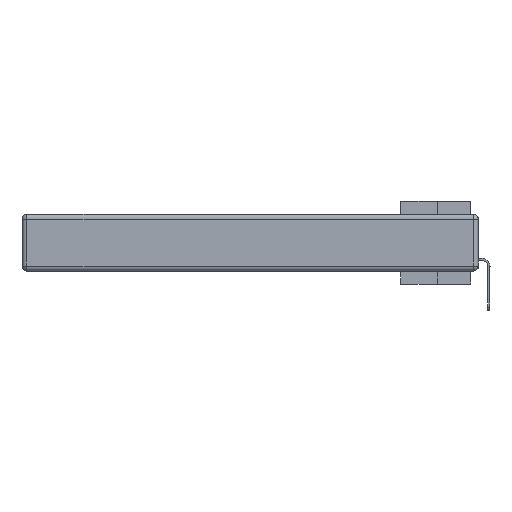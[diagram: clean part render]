
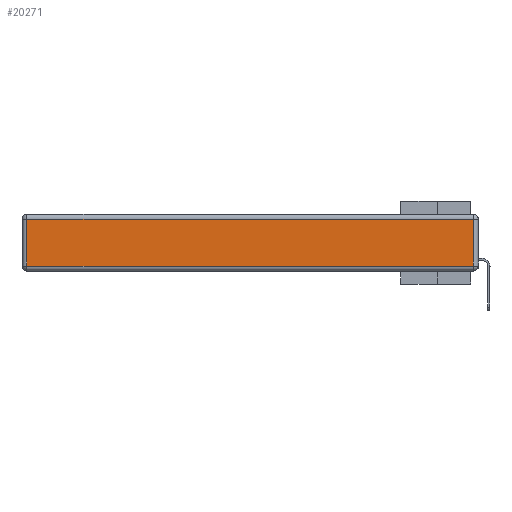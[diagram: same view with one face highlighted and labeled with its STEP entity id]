
A CAD part, left-side view. The second image highlights one B-rep face of the part: STEP entity #20271.
In plain terms, the highlighted planar face has unit normal (-1, 0, 0).
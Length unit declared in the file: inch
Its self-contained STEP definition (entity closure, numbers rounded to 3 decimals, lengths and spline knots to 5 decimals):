
#1172 = VERTEX_POINT ( 'NONE', #33047 ) ;
#1329 = DIRECTION ( 'NONE',  ( 0., 1., 0. ) ) ;
#2897 = EDGE_CURVE ( 'NONE', #21424, #25686, #26747, .T. ) ;
#3691 = VECTOR ( 'NONE', #24142, 39.37008 ) ;
#3718 = CARTESIAN_POINT ( 'NONE',  ( 0., 0.03, -0.343 ) ) ;
#8422 = DIRECTION ( 'NONE',  ( 0., 0., -1. ) ) ;
#8715 = EDGE_CURVE ( 'NONE', #25686, #1172, #25855, .T. ) ;
#9014 = CARTESIAN_POINT ( 'NONE',  ( 0., 0.03, -0.03 ) ) ;
#9244 = ORIENTED_EDGE ( 'NONE', *, *, #13479, .T. ) ;
#9764 = CARTESIAN_POINT ( 'NONE',  ( 0., 2.72, -0.03 ) ) ;
#10135 = DIRECTION ( 'NONE',  ( -1., 0., 0. ) ) ;
#11791 = VERTEX_POINT ( 'NONE', #22369 ) ;
#13479 = EDGE_CURVE ( 'NONE', #1172, #11791, #30309, .T. ) ;
#15377 = ORIENTED_EDGE ( 'NONE', *, *, #8715, .T. ) ;
#16228 = DIRECTION ( 'NONE',  ( 0., -1., 0. ) ) ;
#16686 = ORIENTED_EDGE ( 'NONE', *, *, #23665, .T. ) ;
#16775 = CARTESIAN_POINT ( 'NONE',  ( 0., 2.72, -0.343 ) ) ;
#18112 = PLANE ( 'NONE',  #33064 ) ;
#18398 = LINE ( 'NONE', #3718, #3691 ) ;
#20271 = ADVANCED_FACE ( 'NONE', ( #32194 ), #18112, .T. ) ;
#21080 = CARTESIAN_POINT ( 'NONE',  ( 0., 0., -0.343 ) ) ;
#21424 = VERTEX_POINT ( 'NONE', #9014 ) ;
#22325 = ORIENTED_EDGE ( 'NONE', *, *, #2897, .T. ) ;
#22369 = CARTESIAN_POINT ( 'NONE',  ( 0., 0.03, -0.313 ) ) ;
#23665 = EDGE_CURVE ( 'NONE', #11791, #21424, #18398, .T. ) ;
#24142 = DIRECTION ( 'NONE',  ( 0., 0., 1. ) ) ;
#25386 = VECTOR ( 'NONE', #8422, 39.37008 ) ;
#25686 = VERTEX_POINT ( 'NONE', #9764 ) ;
#25855 = LINE ( 'NONE', #16775, #25386 ) ;
#26088 = VECTOR ( 'NONE', #1329, 39.37008 ) ;
#26642 = EDGE_LOOP ( 'NONE', ( #9244, #16686, #22325, #15377 ) ) ;
#26747 = LINE ( 'NONE', #32510, #26088 ) ;
#29787 = DIRECTION ( 'NONE',  ( 0., 0., 1. ) ) ;
#30309 = LINE ( 'NONE', #31039, #33596 ) ;
#31039 = CARTESIAN_POINT ( 'NONE',  ( 0., 0., -0.313 ) ) ;
#32194 = FACE_OUTER_BOUND ( 'NONE', #26642, .T. ) ;
#32510 = CARTESIAN_POINT ( 'NONE',  ( 0., 2.75, -0.03 ) ) ;
#33047 = CARTESIAN_POINT ( 'NONE',  ( 0., 2.72, -0.313 ) ) ;
#33064 = AXIS2_PLACEMENT_3D ( 'NONE', #21080, #10135, #29787 ) ;
#33596 = VECTOR ( 'NONE', #16228, 39.37008 ) ;
